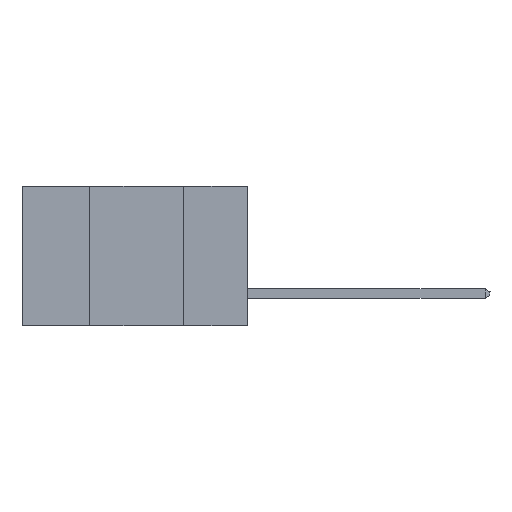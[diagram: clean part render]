
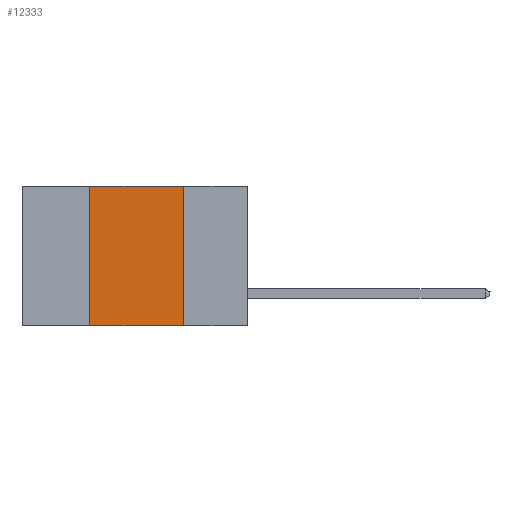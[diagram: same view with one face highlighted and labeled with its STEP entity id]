
A CAD part, left-side view. The second image highlights one B-rep face of the part: STEP entity #12333.
In plain terms, the highlighted planar face has unit normal (-1, 0, 0).
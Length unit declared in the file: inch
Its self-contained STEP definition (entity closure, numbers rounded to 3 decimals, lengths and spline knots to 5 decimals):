
#873 = AXIS2_PLACEMENT_3D ( 'NONE', #4429, #6339, #7347 ) ;
#1129 = VECTOR ( 'NONE', #10834, 39.37008 ) ;
#1195 = VECTOR ( 'NONE', #11763, 39.37008 ) ;
#1590 = VECTOR ( 'NONE', #5661, 39.37008 ) ;
#1957 = ORIENTED_EDGE ( 'NONE', *, *, #9136, .F. ) ;
#3508 = DIRECTION ( 'NONE',  ( 0., -1., 0. ) ) ;
#3733 = CARTESIAN_POINT ( 'NONE',  ( 0., 0.42, 0. ) ) ;
#4291 = EDGE_CURVE ( 'NONE', #7638, #10436, #5602, .T. ) ;
#4429 = CARTESIAN_POINT ( 'NONE',  ( 0., 0.6, 0. ) ) ;
#4498 = FACE_OUTER_BOUND ( 'NONE', #6795, .T. ) ;
#5220 = PLANE ( 'NONE',  #873 ) ;
#5602 = LINE ( 'NONE', #10743, #1590 ) ;
#5661 = DIRECTION ( 'NONE',  ( 0., 0., 1. ) ) ;
#5820 = ORIENTED_EDGE ( 'NONE', *, *, #6139, .F. ) ;
#5874 = LINE ( 'NONE', #8799, #1129 ) ;
#6139 = EDGE_CURVE ( 'NONE', #8567, #10668, #6692, .T. ) ;
#6339 = DIRECTION ( 'NONE',  ( 1., 0., 0. ) ) ;
#6392 = VECTOR ( 'NONE', #3508, 39.37008 ) ;
#6692 = LINE ( 'NONE', #12767, #1195 ) ;
#6795 = EDGE_LOOP ( 'NONE', ( #5820, #1957, #10752, #12671 ) ) ;
#7347 = DIRECTION ( 'NONE',  ( 0., 0., -1. ) ) ;
#7638 = VERTEX_POINT ( 'NONE', #9456 ) ;
#8567 = VERTEX_POINT ( 'NONE', #12446 ) ;
#8799 = CARTESIAN_POINT ( 'NONE',  ( 0., 0.6, 0. ) ) ;
#9079 = EDGE_CURVE ( 'NONE', #7638, #10668, #9524, .T. ) ;
#9136 = EDGE_CURVE ( 'NONE', #10436, #8567, #5874, .T. ) ;
#9456 = CARTESIAN_POINT ( 'NONE',  ( 0., 0.42, -0.37 ) ) ;
#9524 = LINE ( 'NONE', #12565, #6392 ) ;
#10436 = VERTEX_POINT ( 'NONE', #3733 ) ;
#10668 = VERTEX_POINT ( 'NONE', #11681 ) ;
#10743 = CARTESIAN_POINT ( 'NONE',  ( 0., 0.42, -0.37 ) ) ;
#10752 = ORIENTED_EDGE ( 'NONE', *, *, #4291, .F. ) ;
#10834 = DIRECTION ( 'NONE',  ( 0., -1., 0. ) ) ;
#11681 = CARTESIAN_POINT ( 'NONE',  ( 0., 0.17, -0.37 ) ) ;
#11763 = DIRECTION ( 'NONE',  ( 0., 0., -1. ) ) ;
#12333 = ADVANCED_FACE ( 'NONE', ( #4498 ), #5220, .F. ) ;
#12446 = CARTESIAN_POINT ( 'NONE',  ( 0., 0.17, 0. ) ) ;
#12565 = CARTESIAN_POINT ( 'NONE',  ( 0., 0.6, -0.37 ) ) ;
#12671 = ORIENTED_EDGE ( 'NONE', *, *, #9079, .T. ) ;
#12767 = CARTESIAN_POINT ( 'NONE',  ( 0., 0.17, -0.37 ) ) ;
